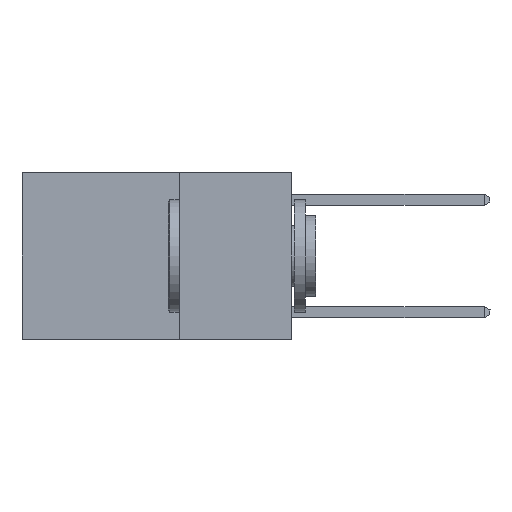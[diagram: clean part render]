
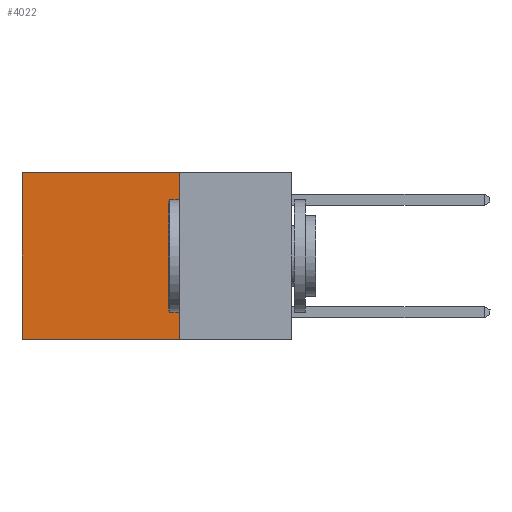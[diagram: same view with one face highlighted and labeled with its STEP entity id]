
A CAD part, left-side view. The second image highlights one B-rep face of the part: STEP entity #4022.
In plain terms, the highlighted planar face has unit normal (-1, 0, 0).
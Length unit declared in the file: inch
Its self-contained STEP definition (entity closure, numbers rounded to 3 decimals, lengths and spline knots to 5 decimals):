
#103 = EDGE_CURVE ( 'NONE', #13938, #2289, #27501, .T. ) ;
#1285 = VECTOR ( 'NONE', #7752, 39.37008 ) ;
#2289 = VERTEX_POINT ( 'NONE', #17985 ) ;
#3703 = PLANE ( 'NONE',  #12864 ) ;
#3983 = DIRECTION ( 'NONE',  ( 0., 1., 0. ) ) ;
#4022 = ADVANCED_FACE ( 'NONE', ( #19320 ), #3703, .F. ) ;
#4194 = EDGE_CURVE ( 'NONE', #2289, #10194, #27767, .T. ) ;
#4762 = EDGE_CURVE ( 'NONE', #19513, #10194, #18134, .T. ) ;
#5126 = CARTESIAN_POINT ( 'NONE',  ( 0.2625, 0.6, -0.37 ) ) ;
#7752 = DIRECTION ( 'NONE',  ( 0., 1., 0. ) ) ;
#9112 = VECTOR ( 'NONE', #26873, 39.37008 ) ;
#9227 = CARTESIAN_POINT ( 'NONE',  ( 0.2625, 0.6, 0. ) ) ;
#10194 = VERTEX_POINT ( 'NONE', #5126 ) ;
#10826 = VECTOR ( 'NONE', #3983, 39.37008 ) ;
#11147 = DIRECTION ( 'NONE',  ( 0., 0., -1. ) ) ;
#12864 = AXIS2_PLACEMENT_3D ( 'NONE', #28209, #25872, #11147 ) ;
#13863 = CARTESIAN_POINT ( 'NONE',  ( 0.2625, 0.25, 0. ) ) ;
#13938 = VERTEX_POINT ( 'NONE', #13863 ) ;
#15293 = ORIENTED_EDGE ( 'NONE', *, *, #103, .T. ) ;
#15641 = LINE ( 'NONE', #19465, #9112 ) ;
#16631 = DIRECTION ( 'NONE',  ( 0., 0., -1. ) ) ;
#17985 = CARTESIAN_POINT ( 'NONE',  ( 0.2625, 0.6, 0. ) ) ;
#18134 = LINE ( 'NONE', #23586, #10826 ) ;
#19320 = FACE_OUTER_BOUND ( 'NONE', #25977, .T. ) ;
#19465 = CARTESIAN_POINT ( 'NONE',  ( 0.2625, 0.25, 0. ) ) ;
#19513 = VERTEX_POINT ( 'NONE', #25550 ) ;
#21247 = VECTOR ( 'NONE', #16631, 39.37008 ) ;
#21491 = ORIENTED_EDGE ( 'NONE', *, *, #30897, .F. ) ;
#23586 = CARTESIAN_POINT ( 'NONE',  ( 0.2625, 0.25, -0.37 ) ) ;
#24134 = ORIENTED_EDGE ( 'NONE', *, *, #4194, .T. ) ;
#24331 = ORIENTED_EDGE ( 'NONE', *, *, #4762, .F. ) ;
#24974 = CARTESIAN_POINT ( 'NONE',  ( 0.2625, 0.25, 0. ) ) ;
#25550 = CARTESIAN_POINT ( 'NONE',  ( 0.2625, 0.25, -0.37 ) ) ;
#25872 = DIRECTION ( 'NONE',  ( 1., 0., 0. ) ) ;
#25977 = EDGE_LOOP ( 'NONE', ( #24134, #24331, #21491, #15293 ) ) ;
#26873 = DIRECTION ( 'NONE',  ( 0., 0., -1. ) ) ;
#27501 = LINE ( 'NONE', #24974, #1285 ) ;
#27767 = LINE ( 'NONE', #9227, #21247 ) ;
#28209 = CARTESIAN_POINT ( 'NONE',  ( 0.2625, 0.25, 0. ) ) ;
#30897 = EDGE_CURVE ( 'NONE', #13938, #19513, #15641, .T. ) ;
